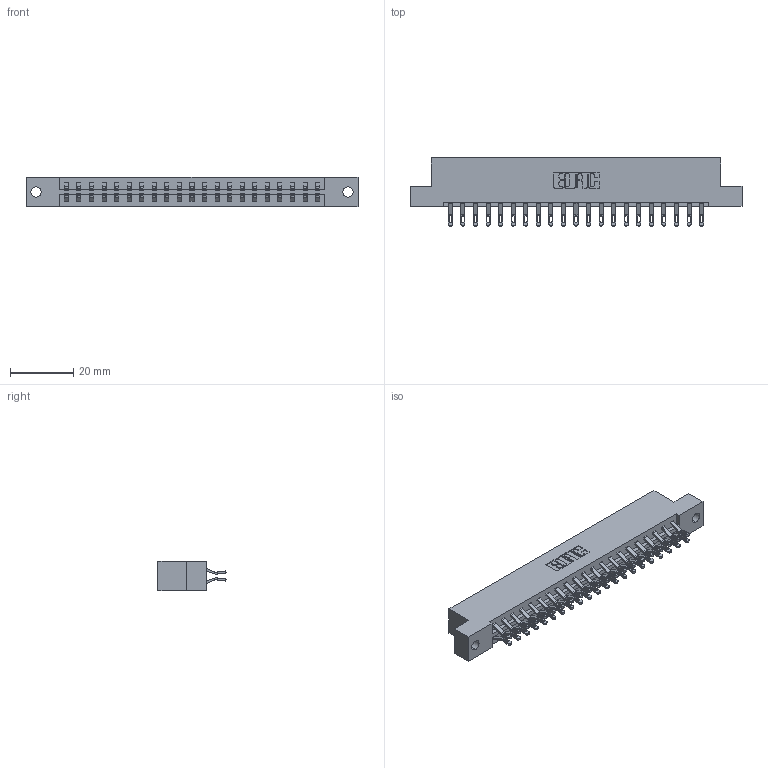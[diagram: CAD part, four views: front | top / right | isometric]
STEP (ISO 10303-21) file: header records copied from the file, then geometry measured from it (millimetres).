
FILE_DESCRIPTION (( 'STEP AP203' ), '1' );
FILE_NAME ('333-042-555-202.STEP', '2018-08-03T19:23:38', ( '' ), ( '' ), 'SwSTEP 2.0', 'SolidWorks 2016', '' );
FILE_SCHEMA (( 'CONFIG_CONTROL_DESIGN' ));
Length unit declared in the file: inch
Products named in the file (3): 333 Part_Flush - .128 Dia; 345-292-001_555 Tail; 333-042-555-202
Assembly tree (43 placements, depth 2):
  333-042-555-202
    333 Part_Flush - .128 Dia
    345-292-001_555 Tail  x42
Bounding box: 104.75 x 21.47 x 9.4 mm (x, y, z)
Volume: 10583.1 mm3; surface area: 12468.5 mm2
Topology: 43 solids, 43 shells, 2550 faces, 7997 edges, 5330 vertices
Faces by surface type: plane 1498, cylinder 1052
Entity records: 16555 total; most frequent: CARTESIAN_POINT 2804, ORIENTED_EDGE 2710, DIRECTION 2403, EDGE_CURVE 1355, VECTOR 1207, LINE 1207, VERTEX_POINT 902, AXIS2_PLACEMENT_3D 598
